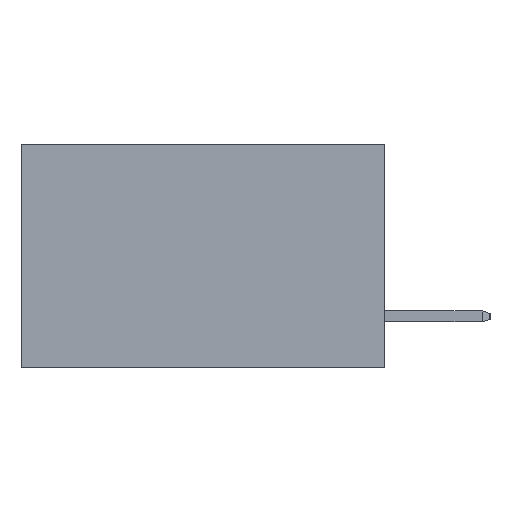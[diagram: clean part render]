
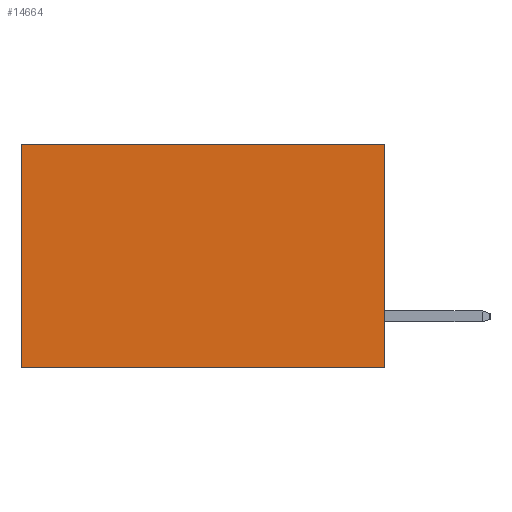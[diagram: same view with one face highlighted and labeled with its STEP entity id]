
A CAD part, left-side view. The second image highlights one B-rep face of the part: STEP entity #14664.
In plain terms, the highlighted planar face has unit normal (-1, 0, 0).
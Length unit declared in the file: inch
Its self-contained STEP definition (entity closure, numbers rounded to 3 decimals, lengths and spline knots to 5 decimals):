
#22 = LINE ( 'NONE', #13446, #15991 ) ;
#533 = CARTESIAN_POINT ( 'NONE',  ( 0.298, 0., 0. ) ) ;
#621 = CARTESIAN_POINT ( 'NONE',  ( 0.298, 0.6, 0. ) ) ;
#876 = CARTESIAN_POINT ( 'NONE',  ( 0.298, 0., 0. ) ) ;
#1118 = LINE ( 'NONE', #621, #13018 ) ;
#1667 = FACE_OUTER_BOUND ( 'NONE', #12179, .T. ) ;
#2504 = DIRECTION ( 'NONE',  ( 1., 0., 0. ) ) ;
#2634 = ORIENTED_EDGE ( 'NONE', *, *, #9290, .T. ) ;
#4978 = CARTESIAN_POINT ( 'NONE',  ( 0.298, 0., -0.37 ) ) ;
#5028 = VERTEX_POINT ( 'NONE', #17014 ) ;
#5111 = EDGE_CURVE ( 'NONE', #8528, #18476, #22, .T. ) ;
#6536 = ORIENTED_EDGE ( 'NONE', *, *, #5111, .F. ) ;
#6742 = ORIENTED_EDGE ( 'NONE', *, *, #16749, .F. ) ;
#7006 = DIRECTION ( 'NONE',  ( 0., 0., -1. ) ) ;
#7534 = VERTEX_POINT ( 'NONE', #15840 ) ;
#8171 = LINE ( 'NONE', #533, #15755 ) ;
#8528 = VERTEX_POINT ( 'NONE', #4978 ) ;
#8646 = DIRECTION ( 'NONE',  ( 0., 1., 0. ) ) ;
#9290 = EDGE_CURVE ( 'NONE', #7534, #5028, #11105, .T. ) ;
#9933 = DIRECTION ( 'NONE',  ( 0., 0., -1. ) ) ;
#11105 = LINE ( 'NONE', #14606, #18695 ) ;
#11801 = PLANE ( 'NONE',  #12308 ) ;
#12179 = EDGE_LOOP ( 'NONE', ( #13103, #6536, #6742, #2634 ) ) ;
#12308 = AXIS2_PLACEMENT_3D ( 'NONE', #876, #2504, #13299 ) ;
#13018 = VECTOR ( 'NONE', #7006, 39.37008 ) ;
#13103 = ORIENTED_EDGE ( 'NONE', *, *, #15891, .T. ) ;
#13299 = DIRECTION ( 'NONE',  ( 0., 0., -1. ) ) ;
#13446 = CARTESIAN_POINT ( 'NONE',  ( 0.298, 0., -0.37 ) ) ;
#14606 = CARTESIAN_POINT ( 'NONE',  ( 0.298, 0., 0. ) ) ;
#14664 = ADVANCED_FACE ( 'NONE', ( #1667 ), #11801, .F. ) ;
#15257 = DIRECTION ( 'NONE',  ( 0., 1., 0. ) ) ;
#15755 = VECTOR ( 'NONE', #9933, 39.37008 ) ;
#15840 = CARTESIAN_POINT ( 'NONE',  ( 0.298, 0., 0. ) ) ;
#15891 = EDGE_CURVE ( 'NONE', #5028, #18476, #1118, .T. ) ;
#15991 = VECTOR ( 'NONE', #15257, 39.37008 ) ;
#16749 = EDGE_CURVE ( 'NONE', #7534, #8528, #8171, .T. ) ;
#17014 = CARTESIAN_POINT ( 'NONE',  ( 0.298, 0.6, 0. ) ) ;
#18476 = VERTEX_POINT ( 'NONE', #19128 ) ;
#18695 = VECTOR ( 'NONE', #8646, 39.37008 ) ;
#19128 = CARTESIAN_POINT ( 'NONE',  ( 0.298, 0.6, -0.37 ) ) ;
